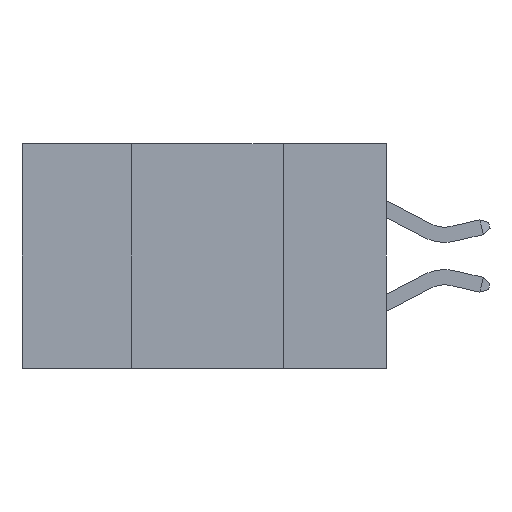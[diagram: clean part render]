
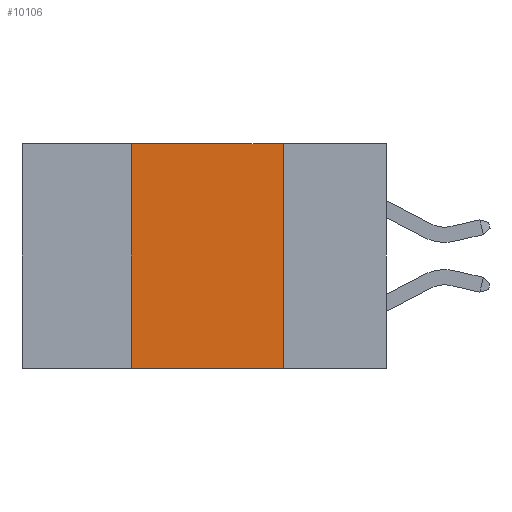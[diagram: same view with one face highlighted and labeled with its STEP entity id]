
A CAD part, left-side view. The second image highlights one B-rep face of the part: STEP entity #10106.
In plain terms, the highlighted planar face has unit normal (-1, 0, 0).
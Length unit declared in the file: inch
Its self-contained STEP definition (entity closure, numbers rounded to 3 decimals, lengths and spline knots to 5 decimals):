
#841 = CARTESIAN_POINT ( 'NONE',  ( 0., 0.42, -0.37 ) ) ;
#1006 = CARTESIAN_POINT ( 'NONE',  ( 0., 0.42, -0.37 ) ) ;
#1489 = ORIENTED_EDGE ( 'NONE', *, *, #8247, .F. ) ;
#1635 = VERTEX_POINT ( 'NONE', #12803 ) ;
#1819 = CARTESIAN_POINT ( 'NONE',  ( 0., 0.6, 0. ) ) ;
#2144 = VECTOR ( 'NONE', #3065, 39.37008 ) ;
#2389 = CARTESIAN_POINT ( 'NONE',  ( 0., 0.42, 0. ) ) ;
#2488 = DIRECTION ( 'NONE',  ( 0., 0., -1. ) ) ;
#3065 = DIRECTION ( 'NONE',  ( 0., -1., 0. ) ) ;
#3814 = EDGE_CURVE ( 'NONE', #4937, #4646, #11110, .T. ) ;
#4153 = VECTOR ( 'NONE', #10391, 39.37008 ) ;
#4444 = CARTESIAN_POINT ( 'NONE',  ( 0., 0.17, -0.37 ) ) ;
#4576 = LINE ( 'NONE', #4444, #6951 ) ;
#4641 = DIRECTION ( 'NONE',  ( 1., 0., 0. ) ) ;
#4646 = VERTEX_POINT ( 'NONE', #13070 ) ;
#4937 = VERTEX_POINT ( 'NONE', #1006 ) ;
#5839 = FACE_OUTER_BOUND ( 'NONE', #6029, .T. ) ;
#5936 = DIRECTION ( 'NONE',  ( 0., 0., 1. ) ) ;
#6002 = LINE ( 'NONE', #841, #6912 ) ;
#6029 = EDGE_LOOP ( 'NONE', ( #10631, #1489, #12672, #10253 ) ) ;
#6703 = PLANE ( 'NONE',  #10096 ) ;
#6840 = DIRECTION ( 'NONE',  ( 0., 0., -1. ) ) ;
#6912 = VECTOR ( 'NONE', #5936, 39.37008 ) ;
#6951 = VECTOR ( 'NONE', #2488, 39.37008 ) ;
#7343 = LINE ( 'NONE', #11389, #4153 ) ;
#8247 = EDGE_CURVE ( 'NONE', #10868, #1635, #7343, .T. ) ;
#9062 = CARTESIAN_POINT ( 'NONE',  ( 0., 0.6, -0.37 ) ) ;
#9838 = EDGE_CURVE ( 'NONE', #4937, #10868, #6002, .T. ) ;
#10096 = AXIS2_PLACEMENT_3D ( 'NONE', #1819, #4641, #6840 ) ;
#10106 = ADVANCED_FACE ( 'NONE', ( #5839 ), #6703, .F. ) ;
#10253 = ORIENTED_EDGE ( 'NONE', *, *, #3814, .T. ) ;
#10391 = DIRECTION ( 'NONE',  ( 0., -1., 0. ) ) ;
#10631 = ORIENTED_EDGE ( 'NONE', *, *, #11906, .F. ) ;
#10868 = VERTEX_POINT ( 'NONE', #2389 ) ;
#11110 = LINE ( 'NONE', #9062, #2144 ) ;
#11389 = CARTESIAN_POINT ( 'NONE',  ( 0., 0.6, 0. ) ) ;
#11906 = EDGE_CURVE ( 'NONE', #1635, #4646, #4576, .T. ) ;
#12672 = ORIENTED_EDGE ( 'NONE', *, *, #9838, .F. ) ;
#12803 = CARTESIAN_POINT ( 'NONE',  ( 0., 0.17, 0. ) ) ;
#13070 = CARTESIAN_POINT ( 'NONE',  ( 0., 0.17, -0.37 ) ) ;
